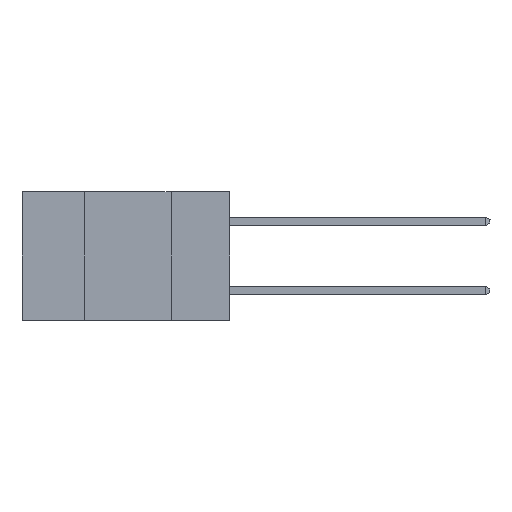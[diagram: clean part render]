
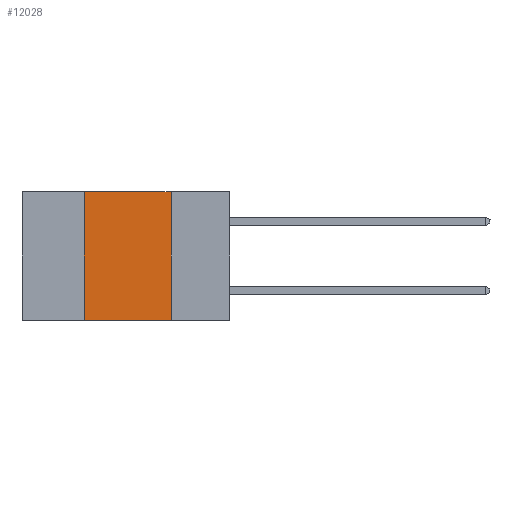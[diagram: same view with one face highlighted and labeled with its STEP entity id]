
A CAD part, left-side view. The second image highlights one B-rep face of the part: STEP entity #12028.
In plain terms, the highlighted planar face has unit normal (-1, 0, 0).
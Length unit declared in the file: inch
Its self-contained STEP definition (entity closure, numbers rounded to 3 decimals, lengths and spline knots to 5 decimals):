
#523 = ORIENTED_EDGE ( 'NONE', *, *, #12751, .F. ) ;
#672 = EDGE_CURVE ( 'NONE', #26184, #17815, #10421, .T. ) ;
#767 = EDGE_LOOP ( 'NONE', ( #15582, #523, #19686, #12300 ) ) ;
#1301 = AXIS2_PLACEMENT_3D ( 'NONE', #8911, #16815, #6538 ) ;
#2538 = CARTESIAN_POINT ( 'NONE',  ( 0., 0.42, -0.37 ) ) ;
#4257 = DIRECTION ( 'NONE',  ( 0., 0., -1. ) ) ;
#4995 = VECTOR ( 'NONE', #14712, 39.37008 ) ;
#5322 = FACE_OUTER_BOUND ( 'NONE', #767, .T. ) ;
#5639 = LINE ( 'NONE', #24534, #4995 ) ;
#5964 = VECTOR ( 'NONE', #4257, 39.37008 ) ;
#6538 = DIRECTION ( 'NONE',  ( 0., 0., -1. ) ) ;
#7842 = CARTESIAN_POINT ( 'NONE',  ( 0., 0.17, -0.37 ) ) ;
#7953 = CARTESIAN_POINT ( 'NONE',  ( 0., 0.42, 0. ) ) ;
#8098 = CARTESIAN_POINT ( 'NONE',  ( 0., 0.17, 0. ) ) ;
#8911 = CARTESIAN_POINT ( 'NONE',  ( 0., 0.6, 0. ) ) ;
#10421 = LINE ( 'NONE', #8098, #5964 ) ;
#12028 = ADVANCED_FACE ( 'NONE', ( #5322 ), #18731, .F. ) ;
#12300 = ORIENTED_EDGE ( 'NONE', *, *, #23231, .T. ) ;
#12751 = EDGE_CURVE ( 'NONE', #17579, #26184, #5639, .T. ) ;
#13198 = LINE ( 'NONE', #20185, #22405 ) ;
#14712 = DIRECTION ( 'NONE',  ( 0., -1., 0. ) ) ;
#14735 = VECTOR ( 'NONE', #22037, 39.37008 ) ;
#15582 = ORIENTED_EDGE ( 'NONE', *, *, #672, .F. ) ;
#16815 = DIRECTION ( 'NONE',  ( 1., 0., 0. ) ) ;
#17579 = VERTEX_POINT ( 'NONE', #7953 ) ;
#17815 = VERTEX_POINT ( 'NONE', #7842 ) ;
#18731 = PLANE ( 'NONE',  #1301 ) ;
#18952 = EDGE_CURVE ( 'NONE', #24100, #17579, #21693, .T. ) ;
#19686 = ORIENTED_EDGE ( 'NONE', *, *, #18952, .F. ) ;
#20185 = CARTESIAN_POINT ( 'NONE',  ( 0., 0.6, -0.37 ) ) ;
#21693 = LINE ( 'NONE', #23801, #14735 ) ;
#22037 = DIRECTION ( 'NONE',  ( 0., 0., 1. ) ) ;
#22154 = CARTESIAN_POINT ( 'NONE',  ( 0., 0.17, 0. ) ) ;
#22405 = VECTOR ( 'NONE', #22476, 39.37008 ) ;
#22476 = DIRECTION ( 'NONE',  ( 0., -1., 0. ) ) ;
#23231 = EDGE_CURVE ( 'NONE', #24100, #17815, #13198, .T. ) ;
#23801 = CARTESIAN_POINT ( 'NONE',  ( 0., 0.42, 0. ) ) ;
#24100 = VERTEX_POINT ( 'NONE', #2538 ) ;
#24534 = CARTESIAN_POINT ( 'NONE',  ( 0., 0.6, 0. ) ) ;
#26184 = VERTEX_POINT ( 'NONE', #22154 ) ;
